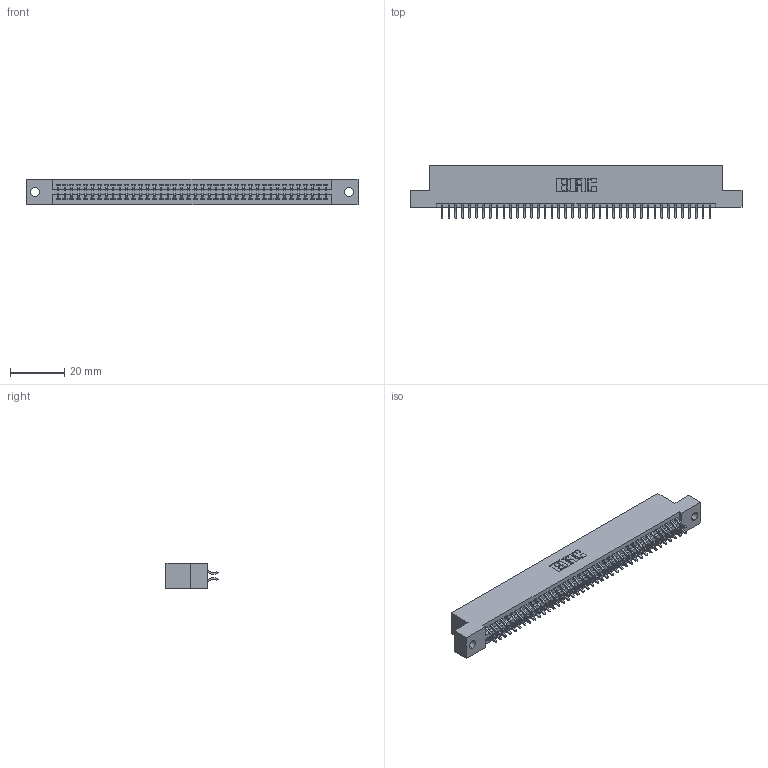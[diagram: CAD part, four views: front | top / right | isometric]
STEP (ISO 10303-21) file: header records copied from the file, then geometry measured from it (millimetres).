
FILE_DESCRIPTION (( 'STEP AP203' ), '1' );
FILE_NAME ('395-080-556-202.STEP', '2018-11-28T05:14:35', ( '' ), ( '' ), 'SwSTEP 2.0', 'SolidWorks 2016', '' );
FILE_SCHEMA (( 'CONFIG_CONTROL_DESIGN' ));
Length unit declared in the file: inch
Products named in the file (3): 395-080-556-202; 345 Part_Flush Mounting Lugs - 0.128 Dia; 345-292-001_556 Tail
Assembly tree (81 placements, depth 2):
  395-080-556-202
    345 Part_Flush Mounting Lugs - 0.128 Dia
    345-292-001_556 Tail  x80
Bounding box: 122.81 x 19.24 x 9.4 mm (x, y, z)
Volume: 11871.4 mm3; surface area: 17166.4 mm2
Topology: 81 solids, 81 shells, 4606 faces, 13701 edges, 9026 vertices
Faces by surface type: plane 3040, cylinder 1566
Entity records: 31877 total; most frequent: CARTESIAN_POINT 5360, ORIENTED_EDGE 5282, DIRECTION 4717, EDGE_CURVE 2641, VECTOR 2341, LINE 2341, VERTEX_POINT 1758, AXIS2_PLACEMENT_3D 1188
